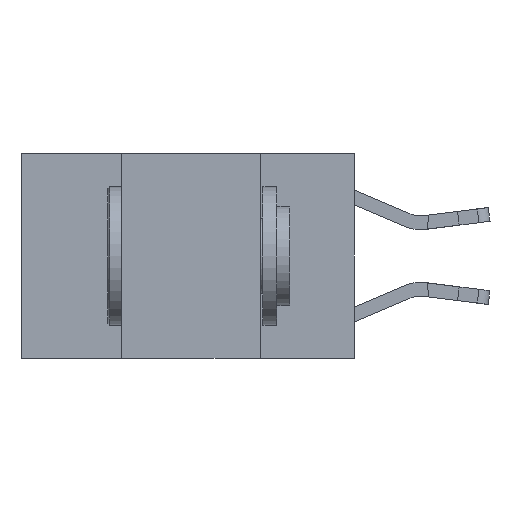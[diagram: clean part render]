
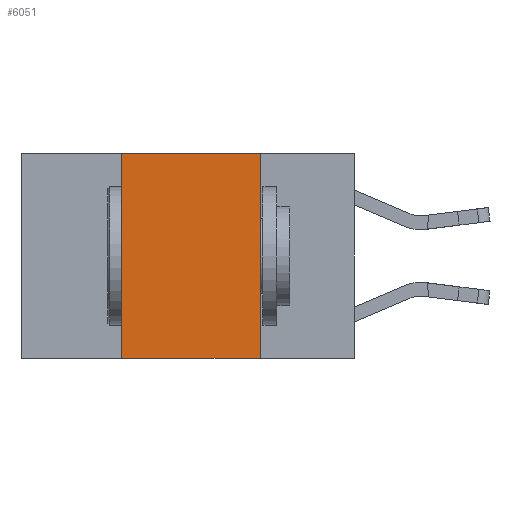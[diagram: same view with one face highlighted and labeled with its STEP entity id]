
A CAD part, left-side view. The second image highlights one B-rep face of the part: STEP entity #6051.
In plain terms, the highlighted planar face has unit normal (-1, 0, 0).
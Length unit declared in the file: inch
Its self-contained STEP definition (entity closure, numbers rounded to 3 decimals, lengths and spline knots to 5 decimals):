
#776 = DIRECTION ( 'NONE',  ( 1., 0., 0. ) ) ;
#839 = PLANE ( 'NONE',  #4040 ) ;
#1449 = DIRECTION ( 'NONE',  ( 0., -1., 0. ) ) ;
#2313 = ORIENTED_EDGE ( 'NONE', *, *, #13102, .F. ) ;
#2902 = VECTOR ( 'NONE', #4236, 39.37008 ) ;
#2915 = EDGE_LOOP ( 'NONE', ( #11703, #12384, #2313, #12421 ) ) ;
#2962 = CARTESIAN_POINT ( 'NONE',  ( 0., 0.42, 0. ) ) ;
#4040 = AXIS2_PLACEMENT_3D ( 'NONE', #12186, #776, #10068 ) ;
#4236 = DIRECTION ( 'NONE',  ( 0., -1., 0. ) ) ;
#4482 = EDGE_CURVE ( 'NONE', #9253, #12221, #11427, .T. ) ;
#4602 = CARTESIAN_POINT ( 'NONE',  ( 0., 0.17, 0. ) ) ;
#4992 = DIRECTION ( 'NONE',  ( 0., 0., 1. ) ) ;
#4997 = CARTESIAN_POINT ( 'NONE',  ( 0., 0.17, -0.37 ) ) ;
#5858 = LINE ( 'NONE', #9570, #10096 ) ;
#6051 = ADVANCED_FACE ( 'NONE', ( #8906 ), #839, .F. ) ;
#6346 = EDGE_CURVE ( 'NONE', #10353, #7731, #5858, .T. ) ;
#6773 = DIRECTION ( 'NONE',  ( 0., 0., -1. ) ) ;
#6914 = VECTOR ( 'NONE', #6773, 39.37008 ) ;
#7411 = LINE ( 'NONE', #4602, #6914 ) ;
#7447 = CARTESIAN_POINT ( 'NONE',  ( 0., 0.42, -0.37 ) ) ;
#7731 = VERTEX_POINT ( 'NONE', #4997 ) ;
#8906 = FACE_OUTER_BOUND ( 'NONE', #2915, .T. ) ;
#9253 = VERTEX_POINT ( 'NONE', #12667 ) ;
#9431 = CARTESIAN_POINT ( 'NONE',  ( 0., 0.6, 0. ) ) ;
#9570 = CARTESIAN_POINT ( 'NONE',  ( 0., 0.6, -0.37 ) ) ;
#9997 = LINE ( 'NONE', #2962, #11310 ) ;
#10026 = EDGE_CURVE ( 'NONE', #12221, #7731, #7411, .T. ) ;
#10068 = DIRECTION ( 'NONE',  ( 0., 0., -1. ) ) ;
#10096 = VECTOR ( 'NONE', #1449, 39.37008 ) ;
#10353 = VERTEX_POINT ( 'NONE', #7447 ) ;
#10366 = CARTESIAN_POINT ( 'NONE',  ( 0., 0.17, 0. ) ) ;
#11310 = VECTOR ( 'NONE', #4992, 39.37008 ) ;
#11427 = LINE ( 'NONE', #9431, #2902 ) ;
#11703 = ORIENTED_EDGE ( 'NONE', *, *, #10026, .F. ) ;
#12186 = CARTESIAN_POINT ( 'NONE',  ( 0., 0.6, 0. ) ) ;
#12221 = VERTEX_POINT ( 'NONE', #10366 ) ;
#12384 = ORIENTED_EDGE ( 'NONE', *, *, #4482, .F. ) ;
#12421 = ORIENTED_EDGE ( 'NONE', *, *, #6346, .T. ) ;
#12667 = CARTESIAN_POINT ( 'NONE',  ( 0., 0.42, 0. ) ) ;
#13102 = EDGE_CURVE ( 'NONE', #10353, #9253, #9997, .T. ) ;
